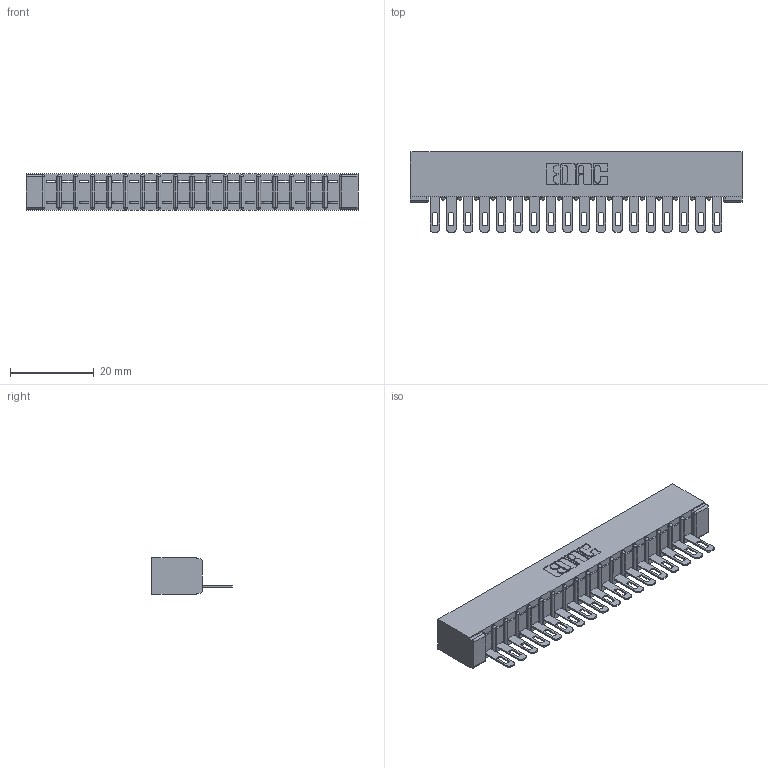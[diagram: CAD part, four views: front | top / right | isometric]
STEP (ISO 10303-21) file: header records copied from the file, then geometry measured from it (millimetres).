
FILE_DESCRIPTION (( 'STEP AP203' ), '1' );
FILE_NAME ('307-018-505-101.STEP', '2019-09-03T17:45:17', ( '' ), ( '' ), 'SwSTEP 2.0', 'SolidWorks 2016', '' );
FILE_SCHEMA (( 'CONFIG_CONTROL_DESIGN' ));
Length unit declared in the file: inch
Products named in the file (3): 307-290-001_505; 307-018-505-101; 307 Part_No Mounting Lugs
Assembly tree (19 placements, depth 2):
  307-018-505-101
    307 Part_No Mounting Lugs
    307-290-001_505  x18
Bounding box: 79.2 x 19.18 x 8.71 mm (x, y, z)
Volume: 5233.2 mm3; surface area: 8420.5 mm2
Topology: 19 solids, 19 shells, 1137 faces, 3215 edges, 2066 vertices
Faces by surface type: plane 714, cylinder 385, sphere 38
Entity records: 18086 total; most frequent: CARTESIAN_POINT 3036, ORIENTED_EDGE 3022, DIRECTION 2967, EDGE_CURVE 1511, LINE 1149, VECTOR 1149, VERTEX_POINT 978, AXIS2_PLACEMENT_3D 909
